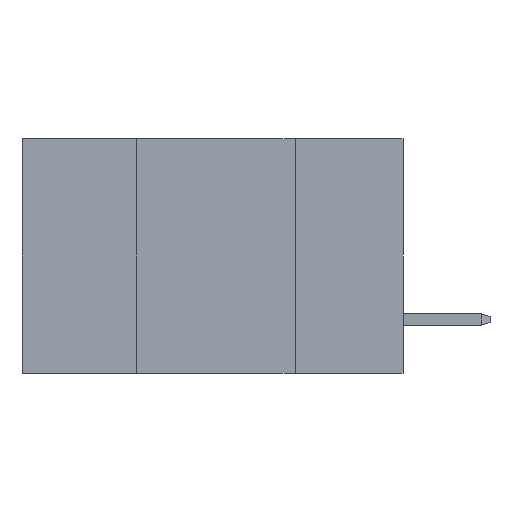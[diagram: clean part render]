
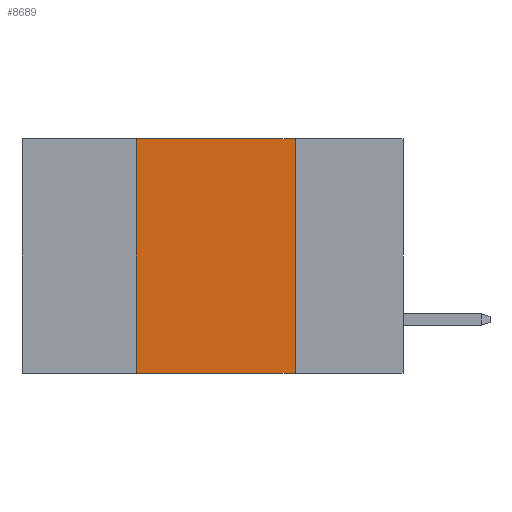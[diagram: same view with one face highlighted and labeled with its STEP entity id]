
A CAD part, left-side view. The second image highlights one B-rep face of the part: STEP entity #8689.
In plain terms, the highlighted planar face has unit normal (-1, 0, 0).
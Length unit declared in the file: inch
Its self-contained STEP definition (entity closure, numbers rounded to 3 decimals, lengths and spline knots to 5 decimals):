
#18 = CARTESIAN_POINT ( 'NONE',  ( 0., 0.42, -0.37 ) ) ;
#123 = ORIENTED_EDGE ( 'NONE', *, *, #2107, .F. ) ;
#496 = EDGE_LOOP ( 'NONE', ( #10704, #6054, #123, #3435 ) ) ;
#694 = EDGE_CURVE ( 'NONE', #6108, #10519, #4073, .T. ) ;
#1642 = CARTESIAN_POINT ( 'NONE',  ( 0., 0.42, 0. ) ) ;
#1696 = DIRECTION ( 'NONE',  ( 0., 0., 1. ) ) ;
#2107 = EDGE_CURVE ( 'NONE', #6108, #4683, #2474, .T. ) ;
#2419 = DIRECTION ( 'NONE',  ( 0., -1., 0. ) ) ;
#2453 = DIRECTION ( 'NONE',  ( 1., 0., 0. ) ) ;
#2474 = LINE ( 'NONE', #1642, #5604 ) ;
#2524 = AXIS2_PLACEMENT_3D ( 'NONE', #9909, #2453, #4934 ) ;
#2564 = VECTOR ( 'NONE', #2419, 39.37008 ) ;
#3435 = ORIENTED_EDGE ( 'NONE', *, *, #694, .T. ) ;
#3493 = LINE ( 'NONE', #5749, #4622 ) ;
#3513 = LINE ( 'NONE', #3572, #4114 ) ;
#3572 = CARTESIAN_POINT ( 'NONE',  ( 0., 0.6, 0. ) ) ;
#4073 = LINE ( 'NONE', #7399, #2564 ) ;
#4114 = VECTOR ( 'NONE', #6036, 39.37008 ) ;
#4169 = DIRECTION ( 'NONE',  ( 0., 0., -1. ) ) ;
#4260 = CARTESIAN_POINT ( 'NONE',  ( 0., 0.42, 0. ) ) ;
#4622 = VECTOR ( 'NONE', #4169, 39.37008 ) ;
#4683 = VERTEX_POINT ( 'NONE', #4260 ) ;
#4934 = DIRECTION ( 'NONE',  ( 0., 0., -1. ) ) ;
#5184 = VERTEX_POINT ( 'NONE', #7849 ) ;
#5604 = VECTOR ( 'NONE', #1696, 39.37008 ) ;
#5671 = EDGE_CURVE ( 'NONE', #5184, #10519, #3493, .T. ) ;
#5749 = CARTESIAN_POINT ( 'NONE',  ( 0., 0.17, 0. ) ) ;
#6036 = DIRECTION ( 'NONE',  ( 0., -1., 0. ) ) ;
#6054 = ORIENTED_EDGE ( 'NONE', *, *, #8367, .F. ) ;
#6108 = VERTEX_POINT ( 'NONE', #18 ) ;
#7399 = CARTESIAN_POINT ( 'NONE',  ( 0., 0.6, -0.37 ) ) ;
#7446 = FACE_OUTER_BOUND ( 'NONE', #496, .T. ) ;
#7849 = CARTESIAN_POINT ( 'NONE',  ( 0., 0.17, 0. ) ) ;
#8327 = PLANE ( 'NONE',  #2524 ) ;
#8367 = EDGE_CURVE ( 'NONE', #4683, #5184, #3513, .T. ) ;
#8689 = ADVANCED_FACE ( 'NONE', ( #7446 ), #8327, .F. ) ;
#8872 = CARTESIAN_POINT ( 'NONE',  ( 0., 0.17, -0.37 ) ) ;
#9909 = CARTESIAN_POINT ( 'NONE',  ( 0., 0.6, 0. ) ) ;
#10519 = VERTEX_POINT ( 'NONE', #8872 ) ;
#10704 = ORIENTED_EDGE ( 'NONE', *, *, #5671, .F. ) ;
